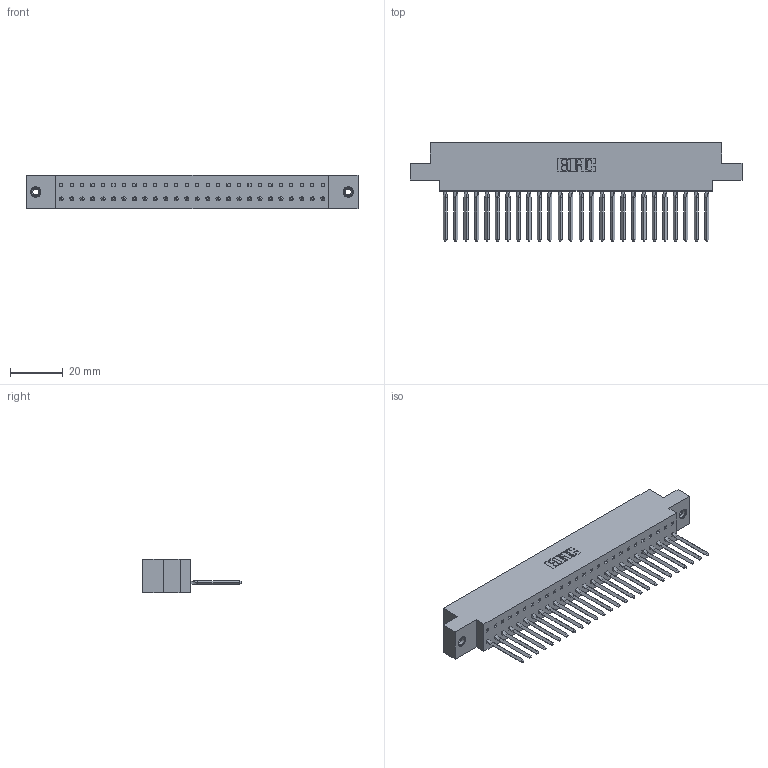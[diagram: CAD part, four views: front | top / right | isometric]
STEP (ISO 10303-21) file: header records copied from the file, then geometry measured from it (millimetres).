
FILE_DESCRIPTION (( 'STEP AP203' ), '1' );
FILE_NAME ('317-026-541-608.STEP', '2020-02-27T18:45:20', ( '' ), ( '' ), 'SwSTEP 2.0', 'SolidWorks 2016', '' );
FILE_SCHEMA (( 'CONFIG_CONTROL_DESIGN' ));
Length unit declared in the file: inch
Products named in the file (4): 345-250-001_345-250-003-102; 317 Part_.156 Dia - TI; 317-290-002_541; 317-026-541-608
Assembly tree (29 placements, depth 2):
  317-026-541-608
    317 Part_.156 Dia - TI
    317-290-002_541  x26
    345-250-001_345-250-003-102  x2
Bounding box: 125.73 x 37.34 x 12.7 mm (x, y, z)
Volume: 19890.7 mm3; surface area: 27595 mm2
Topology: 29 solids, 29 shells, 4114 faces, 11695 edges, 7598 vertices
Faces by surface type: plane 3314, cylinder 680, bspline 104, cone 12, torus 4
Entity records: 41717 total; most frequent: CARTESIAN_POINT 8018, ORIENTED_EDGE 7290, DIRECTION 6019, EDGE_CURVE 3645, LINE 3261, VECTOR 3261, VERTEX_POINT 2418, AXIS2_PLACEMENT_3D 1379
